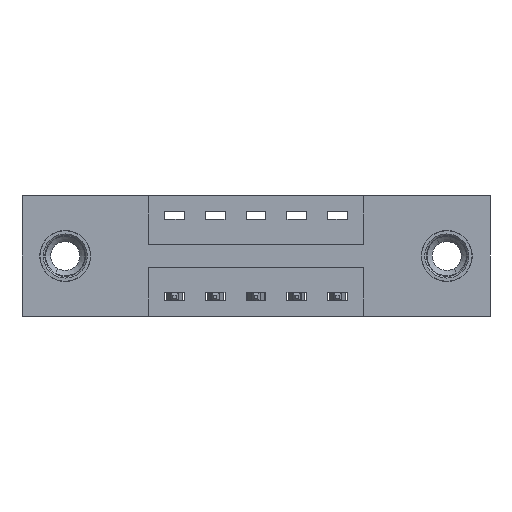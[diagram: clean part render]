
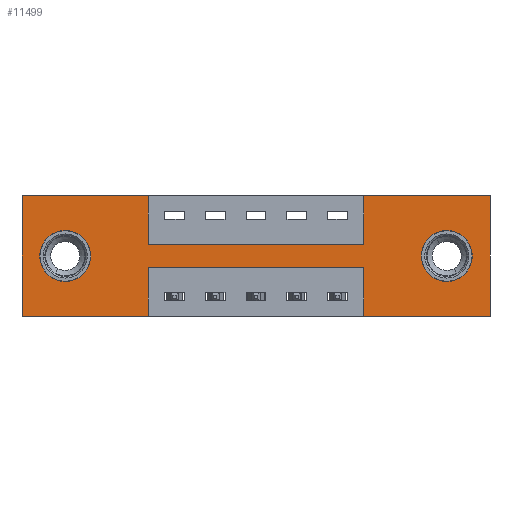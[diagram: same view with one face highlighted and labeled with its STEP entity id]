
A CAD part, front view. The second image highlights one B-rep face of the part: STEP entity #11499.
In plain terms, the highlighted planar face has unit normal (0, -1, 0).
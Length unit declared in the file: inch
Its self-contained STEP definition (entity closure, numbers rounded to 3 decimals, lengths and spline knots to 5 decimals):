
#37 = VERTEX_POINT ( 'NONE', #4060 ) ;
#76 = CARTESIAN_POINT ( 'NONE',  ( 1.435, 0., 0. ) ) ;
#192 = VECTOR ( 'NONE', #1788, 39.37008 ) ;
#199 = VECTOR ( 'NONE', #4944, 39.37008 ) ;
#344 = ORIENTED_EDGE ( 'NONE', *, *, #9415, .F. ) ;
#439 = ORIENTED_EDGE ( 'NONE', *, *, #8626, .T. ) ;
#577 = DIRECTION ( 'NONE',  ( -1., 0., 0. ) ) ;
#675 = VERTEX_POINT ( 'NONE', #7239 ) ;
#725 = AXIS2_PLACEMENT_3D ( 'NONE', #2236, #8183, #1223 ) ;
#739 = CARTESIAN_POINT ( 'NONE',  ( 1.435, 0., -0.37 ) ) ;
#752 = LINE ( 'NONE', #12194, #2466 ) ;
#760 = CARTESIAN_POINT ( 'NONE',  ( 1.0475, 0., 0. ) ) ;
#768 = FACE_BOUND ( 'NONE', #8707, .T. ) ;
#998 = CARTESIAN_POINT ( 'NONE',  ( 0.3875, 0., -0.15 ) ) ;
#1193 = VERTEX_POINT ( 'NONE', #76 ) ;
#1206 = VECTOR ( 'NONE', #11116, 39.37008 ) ;
#1223 = DIRECTION ( 'NONE',  ( 0., 0., 1. ) ) ;
#1331 = CARTESIAN_POINT ( 'NONE',  ( 0.3875, 0., -0.15 ) ) ;
#1478 = VECTOR ( 'NONE', #577, 39.37008 ) ;
#1517 = LINE ( 'NONE', #8036, #1206 ) ;
#1529 = VERTEX_POINT ( 'NONE', #6502 ) ;
#1566 = DIRECTION ( 'NONE',  ( 0., 1., 0. ) ) ;
#1632 = VERTEX_POINT ( 'NONE', #739 ) ;
#1633 = PLANE ( 'NONE',  #4559 ) ;
#1741 = ORIENTED_EDGE ( 'NONE', *, *, #8811, .F. ) ;
#1788 = DIRECTION ( 'NONE',  ( 0., 0., 1. ) ) ;
#2033 = LINE ( 'NONE', #760, #192 ) ;
#2225 = VECTOR ( 'NONE', #4059, 39.37008 ) ;
#2236 = CARTESIAN_POINT ( 'NONE',  ( 0.1325, 0., -0.185 ) ) ;
#2272 = ORIENTED_EDGE ( 'NONE', *, *, #4076, .F. ) ;
#2317 = EDGE_CURVE ( 'NONE', #2638, #5706, #7273, .T. ) ;
#2334 = DIRECTION ( 'NONE',  ( -1., 0., 0. ) ) ;
#2435 = CARTESIAN_POINT ( 'NONE',  ( 0., 0., 0. ) ) ;
#2466 = VECTOR ( 'NONE', #2334, 39.37008 ) ;
#2470 = DIRECTION ( 'NONE',  ( 0., 0., -1. ) ) ;
#2593 = LINE ( 'NONE', #12672, #4262 ) ;
#2627 = FACE_OUTER_BOUND ( 'NONE', #7861, .T. ) ;
#2638 = VERTEX_POINT ( 'NONE', #12436 ) ;
#2646 = EDGE_CURVE ( 'NONE', #37, #675, #12474, .T. ) ;
#2647 = CARTESIAN_POINT ( 'NONE',  ( 0., 0., -0.37 ) ) ;
#3067 = LINE ( 'NONE', #998, #5730 ) ;
#3398 = CARTESIAN_POINT ( 'NONE',  ( 1.3025, 0., -0.185 ) ) ;
#3455 = VERTEX_POINT ( 'NONE', #5324 ) ;
#3459 = ORIENTED_EDGE ( 'NONE', *, *, #6832, .F. ) ;
#3527 = ORIENTED_EDGE ( 'NONE', *, *, #11558, .F. ) ;
#3569 = CARTESIAN_POINT ( 'NONE',  ( 1.3025, 0., -0.185 ) ) ;
#3633 = EDGE_CURVE ( 'NONE', #3455, #6801, #6546, .T. ) ;
#3721 = CARTESIAN_POINT ( 'NONE',  ( 0.1325, 0., -0.185 ) ) ;
#3873 = VECTOR ( 'NONE', #6235, 39.37008 ) ;
#4042 = AXIS2_PLACEMENT_3D ( 'NONE', #3398, #6404, #7332 ) ;
#4059 = DIRECTION ( 'NONE',  ( 0., 0., -1. ) ) ;
#4060 = CARTESIAN_POINT ( 'NONE',  ( 0.1325, 0., -0.263 ) ) ;
#4076 = EDGE_CURVE ( 'NONE', #5706, #8008, #2593, .T. ) ;
#4080 = VECTOR ( 'NONE', #9270, 39.37008 ) ;
#4159 = CIRCLE ( 'NONE', #4042, 0.078 ) ;
#4180 = CARTESIAN_POINT ( 'NONE',  ( 0., 0., -0.37 ) ) ;
#4262 = VECTOR ( 'NONE', #9773, 39.37008 ) ;
#4406 = ORIENTED_EDGE ( 'NONE', *, *, #6749, .F. ) ;
#4444 = CARTESIAN_POINT ( 'NONE',  ( 1.3025, 0., -0.107 ) ) ;
#4559 = AXIS2_PLACEMENT_3D ( 'NONE', #2647, #11562, #12645 ) ;
#4716 = EDGE_CURVE ( 'NONE', #1193, #1632, #9410, .T. ) ;
#4719 = DIRECTION ( 'NONE',  ( 0., 0., 1. ) ) ;
#4777 = ORIENTED_EDGE ( 'NONE', *, *, #4716, .F. ) ;
#4944 = DIRECTION ( 'NONE',  ( 1., 0., 0. ) ) ;
#5324 = CARTESIAN_POINT ( 'NONE',  ( 1.0475, 0., -0.37 ) ) ;
#5326 = VERTEX_POINT ( 'NONE', #5590 ) ;
#5491 = AXIS2_PLACEMENT_3D ( 'NONE', #3569, #1566, #8718 ) ;
#5552 = ORIENTED_EDGE ( 'NONE', *, *, #7652, .F. ) ;
#5590 = CARTESIAN_POINT ( 'NONE',  ( 0., 0., -0.37 ) ) ;
#5706 = VERTEX_POINT ( 'NONE', #8706 ) ;
#5730 = VECTOR ( 'NONE', #8639, 39.37008 ) ;
#6235 = DIRECTION ( 'NONE',  ( -1., 0., 0. ) ) ;
#6404 = DIRECTION ( 'NONE',  ( 0., 1., 0. ) ) ;
#6434 = CARTESIAN_POINT ( 'NONE',  ( 0., 0., 0. ) ) ;
#6502 = CARTESIAN_POINT ( 'NONE',  ( 0.3875, 0., -0.22 ) ) ;
#6546 = LINE ( 'NONE', #8150, #9942 ) ;
#6581 = VERTEX_POINT ( 'NONE', #11967 ) ;
#6598 = ORIENTED_EDGE ( 'NONE', *, *, #8057, .F. ) ;
#6722 = FACE_BOUND ( 'NONE', #12336, .T. ) ;
#6749 = EDGE_CURVE ( 'NONE', #6581, #5326, #752, .T. ) ;
#6801 = VERTEX_POINT ( 'NONE', #12325 ) ;
#6832 = EDGE_CURVE ( 'NONE', #8008, #7669, #3067, .T. ) ;
#7104 = CARTESIAN_POINT ( 'NONE',  ( 1.3025, 0., -0.263 ) ) ;
#7121 = CARTESIAN_POINT ( 'NONE',  ( 0.3875, 0., -0.37 ) ) ;
#7165 = ORIENTED_EDGE ( 'NONE', *, *, #3633, .F. ) ;
#7239 = CARTESIAN_POINT ( 'NONE',  ( 0.1325, 0., -0.107 ) ) ;
#7273 = LINE ( 'NONE', #6434, #199 ) ;
#7332 = DIRECTION ( 'NONE',  ( 0., 0., -1. ) ) ;
#7479 = ORIENTED_EDGE ( 'NONE', *, *, #2646, .T. ) ;
#7652 = EDGE_CURVE ( 'NONE', #6801, #1529, #11773, .T. ) ;
#7669 = VERTEX_POINT ( 'NONE', #7684 ) ;
#7684 = CARTESIAN_POINT ( 'NONE',  ( 1.0475, 0., -0.15 ) ) ;
#7861 = EDGE_LOOP ( 'NONE', ( #1741, #5552, #7165, #344, #4777, #6598, #11931, #3459, #2272, #9062, #3527, #4406 ) ) ;
#7915 = VERTEX_POINT ( 'NONE', #7104 ) ;
#8008 = VERTEX_POINT ( 'NONE', #1331 ) ;
#8036 = CARTESIAN_POINT ( 'NONE',  ( 0., 0., 0. ) ) ;
#8057 = EDGE_CURVE ( 'NONE', #10651, #1193, #12517, .T. ) ;
#8150 = CARTESIAN_POINT ( 'NONE',  ( 1.0475, 0., -0.37 ) ) ;
#8183 = DIRECTION ( 'NONE',  ( 0., 1., 0. ) ) ;
#8479 = CARTESIAN_POINT ( 'NONE',  ( 1.435, 0., 0. ) ) ;
#8556 = EDGE_CURVE ( 'NONE', #675, #37, #11114, .T. ) ;
#8559 = CARTESIAN_POINT ( 'NONE',  ( 1.0475, 0., 0. ) ) ;
#8626 = EDGE_CURVE ( 'NONE', #12533, #7915, #12503, .T. ) ;
#8639 = DIRECTION ( 'NONE',  ( 1., 0., 0. ) ) ;
#8706 = CARTESIAN_POINT ( 'NONE',  ( 0.3875, 0., 0. ) ) ;
#8707 = EDGE_LOOP ( 'NONE', ( #8753, #7479 ) ) ;
#8718 = DIRECTION ( 'NONE',  ( 0., 0., -1. ) ) ;
#8753 = ORIENTED_EDGE ( 'NONE', *, *, #8556, .T. ) ;
#8811 = EDGE_CURVE ( 'NONE', #1529, #6581, #9246, .T. ) ;
#8833 = VECTOR ( 'NONE', #2470, 39.37008 ) ;
#8993 = DIRECTION ( 'NONE',  ( 0., 0., 1. ) ) ;
#9062 = ORIENTED_EDGE ( 'NONE', *, *, #2317, .F. ) ;
#9088 = LINE ( 'NONE', #4180, #3873 ) ;
#9233 = EDGE_CURVE ( 'NONE', #7669, #10651, #2033, .T. ) ;
#9246 = LINE ( 'NONE', #7121, #2225 ) ;
#9270 = DIRECTION ( 'NONE',  ( 1., 0., 0. ) ) ;
#9410 = LINE ( 'NONE', #8479, #8833 ) ;
#9415 = EDGE_CURVE ( 'NONE', #1632, #3455, #9088, .T. ) ;
#9773 = DIRECTION ( 'NONE',  ( 0., 0., -1. ) ) ;
#9942 = VECTOR ( 'NONE', #8993, 39.37008 ) ;
#10214 = EDGE_CURVE ( 'NONE', #7915, #12533, #4159, .T. ) ;
#10651 = VERTEX_POINT ( 'NONE', #8559 ) ;
#10715 = DIRECTION ( 'NONE',  ( 0., 1., 0. ) ) ;
#10939 = AXIS2_PLACEMENT_3D ( 'NONE', #3721, #10715, #4719 ) ;
#11114 = CIRCLE ( 'NONE', #725, 0.078 ) ;
#11116 = DIRECTION ( 'NONE',  ( 0., 0., 1. ) ) ;
#11499 = ADVANCED_FACE ( 'NONE', ( #6722, #768, #2627 ), #1633, .T. ) ;
#11558 = EDGE_CURVE ( 'NONE', #5326, #2638, #1517, .T. ) ;
#11562 = DIRECTION ( 'NONE',  ( 0., -1., 0. ) ) ;
#11773 = LINE ( 'NONE', #12529, #1478 ) ;
#11931 = ORIENTED_EDGE ( 'NONE', *, *, #9233, .F. ) ;
#11967 = CARTESIAN_POINT ( 'NONE',  ( 0.3875, 0., -0.37 ) ) ;
#11969 = ORIENTED_EDGE ( 'NONE', *, *, #10214, .T. ) ;
#12194 = CARTESIAN_POINT ( 'NONE',  ( 0., 0., -0.37 ) ) ;
#12325 = CARTESIAN_POINT ( 'NONE',  ( 1.0475, 0., -0.22 ) ) ;
#12336 = EDGE_LOOP ( 'NONE', ( #439, #11969 ) ) ;
#12436 = CARTESIAN_POINT ( 'NONE',  ( 0., 0., 0. ) ) ;
#12474 = CIRCLE ( 'NONE', #10939, 0.078 ) ;
#12503 = CIRCLE ( 'NONE', #5491, 0.078 ) ;
#12517 = LINE ( 'NONE', #2435, #4080 ) ;
#12529 = CARTESIAN_POINT ( 'NONE',  ( 0.3875, 0., -0.22 ) ) ;
#12533 = VERTEX_POINT ( 'NONE', #4444 ) ;
#12645 = DIRECTION ( 'NONE',  ( 0., 0., -1. ) ) ;
#12672 = CARTESIAN_POINT ( 'NONE',  ( 0.3875, 0., 0. ) ) ;
